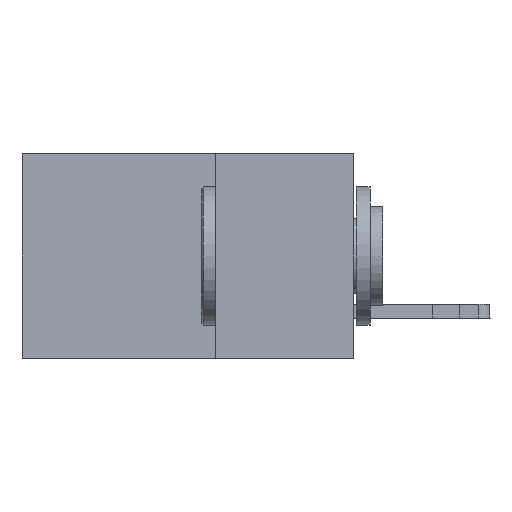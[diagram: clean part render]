
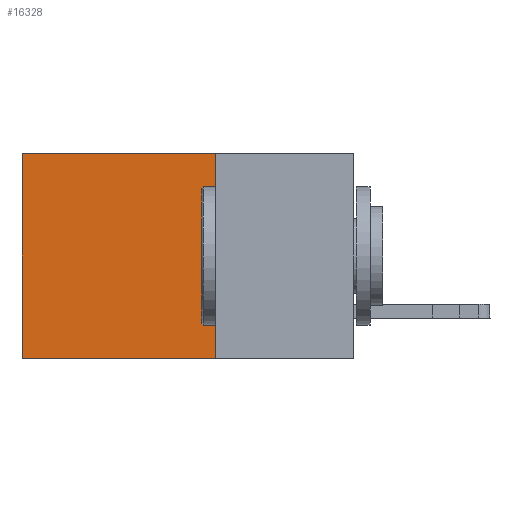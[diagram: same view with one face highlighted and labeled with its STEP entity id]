
A CAD part, left-side view. The second image highlights one B-rep face of the part: STEP entity #16328.
In plain terms, the highlighted planar face has unit normal (-1, 0, 0).
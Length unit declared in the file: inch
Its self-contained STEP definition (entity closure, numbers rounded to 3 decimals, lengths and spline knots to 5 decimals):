
#851 = CARTESIAN_POINT ( 'NONE',  ( 0.2875, 0.25, 0. ) ) ;
#974 = ORIENTED_EDGE ( 'NONE', *, *, #16129, .T. ) ;
#1162 = LINE ( 'NONE', #19674, #15889 ) ;
#1931 = CARTESIAN_POINT ( 'NONE',  ( 0.2875, 0.25, 0. ) ) ;
#2112 = DIRECTION ( 'NONE',  ( 0., 0., -1. ) ) ;
#2611 = EDGE_LOOP ( 'NONE', ( #974, #9188, #5285, #7224 ) ) ;
#2730 = VERTEX_POINT ( 'NONE', #21894 ) ;
#3055 = EDGE_CURVE ( 'NONE', #17854, #23376, #19593, .T. ) ;
#3321 = VECTOR ( 'NONE', #10947, 39.37008 ) ;
#4178 = FACE_OUTER_BOUND ( 'NONE', #2611, .T. ) ;
#4964 = EDGE_CURVE ( 'NONE', #2730, #5108, #1162, .T. ) ;
#5108 = VERTEX_POINT ( 'NONE', #14367 ) ;
#5285 = ORIENTED_EDGE ( 'NONE', *, *, #8692, .F. ) ;
#7224 = ORIENTED_EDGE ( 'NONE', *, *, #3055, .T. ) ;
#8692 = EDGE_CURVE ( 'NONE', #17854, #2730, #16594, .T. ) ;
#9188 = ORIENTED_EDGE ( 'NONE', *, *, #4964, .F. ) ;
#9681 = PLANE ( 'NONE',  #16463 ) ;
#10947 = DIRECTION ( 'NONE',  ( 0., 0., -1. ) ) ;
#11389 = DIRECTION ( 'NONE',  ( 0., 1., 0. ) ) ;
#13541 = DIRECTION ( 'NONE',  ( 1., 0., 0. ) ) ;
#13874 = VECTOR ( 'NONE', #11389, 39.37008 ) ;
#14367 = CARTESIAN_POINT ( 'NONE',  ( 0.2875, 0.6, -0.37 ) ) ;
#15341 = DIRECTION ( 'NONE',  ( 0., 0., -1. ) ) ;
#15889 = VECTOR ( 'NONE', #21600, 39.37008 ) ;
#16129 = EDGE_CURVE ( 'NONE', #23376, #5108, #24277, .T. ) ;
#16328 = ADVANCED_FACE ( 'NONE', ( #4178 ), #9681, .F. ) ;
#16463 = AXIS2_PLACEMENT_3D ( 'NONE', #23095, #13541, #2112 ) ;
#16594 = LINE ( 'NONE', #1931, #21025 ) ;
#16731 = CARTESIAN_POINT ( 'NONE',  ( 0.2875, 0.6, 0. ) ) ;
#17854 = VERTEX_POINT ( 'NONE', #851 ) ;
#19593 = LINE ( 'NONE', #24792, #13874 ) ;
#19674 = CARTESIAN_POINT ( 'NONE',  ( 0.2875, 0.25, -0.37 ) ) ;
#21025 = VECTOR ( 'NONE', #15341, 39.37008 ) ;
#21600 = DIRECTION ( 'NONE',  ( 0., 1., 0. ) ) ;
#21894 = CARTESIAN_POINT ( 'NONE',  ( 0.2875, 0.25, -0.37 ) ) ;
#23095 = CARTESIAN_POINT ( 'NONE',  ( 0.2875, 0.25, 0. ) ) ;
#23376 = VERTEX_POINT ( 'NONE', #24732 ) ;
#24277 = LINE ( 'NONE', #16731, #3321 ) ;
#24732 = CARTESIAN_POINT ( 'NONE',  ( 0.2875, 0.6, 0. ) ) ;
#24792 = CARTESIAN_POINT ( 'NONE',  ( 0.2875, 0.25, 0. ) ) ;
